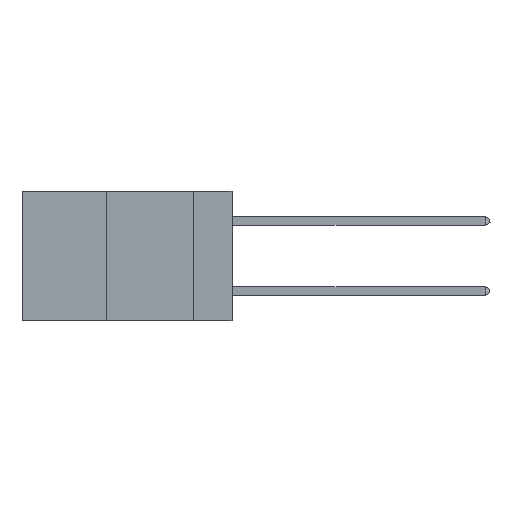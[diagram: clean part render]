
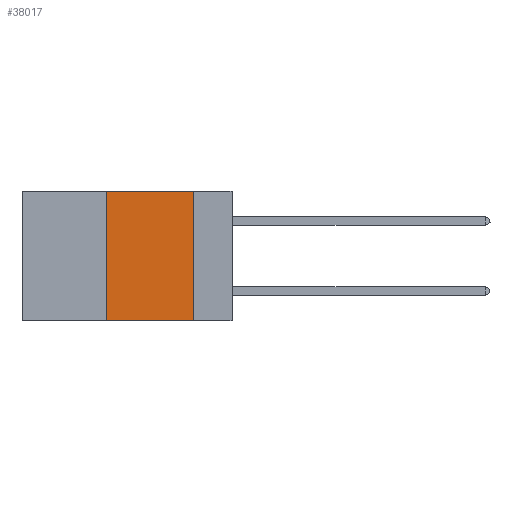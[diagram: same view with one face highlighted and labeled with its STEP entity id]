
A CAD part, left-side view. The second image highlights one B-rep face of the part: STEP entity #38017.
In plain terms, the highlighted planar face has unit normal (-1, 0, 0).
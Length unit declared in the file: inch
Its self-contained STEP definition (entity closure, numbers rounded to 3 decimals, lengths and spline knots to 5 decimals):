
#456 = LINE ( 'NONE', #3629, #20171 ) ;
#2144 = CARTESIAN_POINT ( 'NONE',  ( 0., 0.11, -0.37 ) ) ;
#2915 = CARTESIAN_POINT ( 'NONE',  ( 0., 0.36, -0.37 ) ) ;
#3629 = CARTESIAN_POINT ( 'NONE',  ( 0., 0.6, -0.37 ) ) ;
#4590 = CARTESIAN_POINT ( 'NONE',  ( 0., 0.11, 0. ) ) ;
#5665 = ORIENTED_EDGE ( 'NONE', *, *, #6912, .F. ) ;
#6175 = CARTESIAN_POINT ( 'NONE',  ( 0., 0.11, 0. ) ) ;
#6550 = EDGE_LOOP ( 'NONE', ( #34701, #21179, #5665, #43548 ) ) ;
#6912 = EDGE_CURVE ( 'NONE', #21945, #45028, #35756, .T. ) ;
#7075 = DIRECTION ( 'NONE',  ( 1., 0., 0. ) ) ;
#8560 = FACE_OUTER_BOUND ( 'NONE', #6550, .T. ) ;
#8809 = DIRECTION ( 'NONE',  ( 0., 0., 1. ) ) ;
#8834 = CARTESIAN_POINT ( 'NONE',  ( 0., 0.36, 0. ) ) ;
#10624 = PLANE ( 'NONE',  #35977 ) ;
#13055 = DIRECTION ( 'NONE',  ( 0., 0., -1. ) ) ;
#13321 = LINE ( 'NONE', #28873, #46789 ) ;
#14969 = EDGE_CURVE ( 'NONE', #21861, #19764, #17211, .T. ) ;
#16106 = CARTESIAN_POINT ( 'NONE',  ( 0., 0.36, 0. ) ) ;
#16177 = VECTOR ( 'NONE', #8809, 39.37008 ) ;
#16604 = EDGE_CURVE ( 'NONE', #21945, #19764, #456, .T. ) ;
#17211 = LINE ( 'NONE', #4590, #45473 ) ;
#19764 = VERTEX_POINT ( 'NONE', #2144 ) ;
#20171 = VECTOR ( 'NONE', #40793, 39.37008 ) ;
#21179 = ORIENTED_EDGE ( 'NONE', *, *, #22359, .F. ) ;
#21861 = VERTEX_POINT ( 'NONE', #6175 ) ;
#21916 = DIRECTION ( 'NONE',  ( 0., 0., -1. ) ) ;
#21945 = VERTEX_POINT ( 'NONE', #2915 ) ;
#22359 = EDGE_CURVE ( 'NONE', #45028, #21861, #13321, .T. ) ;
#24843 = DIRECTION ( 'NONE',  ( 0., -1., 0. ) ) ;
#28873 = CARTESIAN_POINT ( 'NONE',  ( 0., 0.6, 0. ) ) ;
#29312 = CARTESIAN_POINT ( 'NONE',  ( 0., 0.6, 0. ) ) ;
#34701 = ORIENTED_EDGE ( 'NONE', *, *, #14969, .F. ) ;
#35756 = LINE ( 'NONE', #16106, #16177 ) ;
#35977 = AXIS2_PLACEMENT_3D ( 'NONE', #29312, #7075, #21916 ) ;
#38017 = ADVANCED_FACE ( 'NONE', ( #8560 ), #10624, .F. ) ;
#40793 = DIRECTION ( 'NONE',  ( 0., -1., 0. ) ) ;
#43548 = ORIENTED_EDGE ( 'NONE', *, *, #16604, .T. ) ;
#45028 = VERTEX_POINT ( 'NONE', #8834 ) ;
#45473 = VECTOR ( 'NONE', #13055, 39.37008 ) ;
#46789 = VECTOR ( 'NONE', #24843, 39.37008 ) ;
